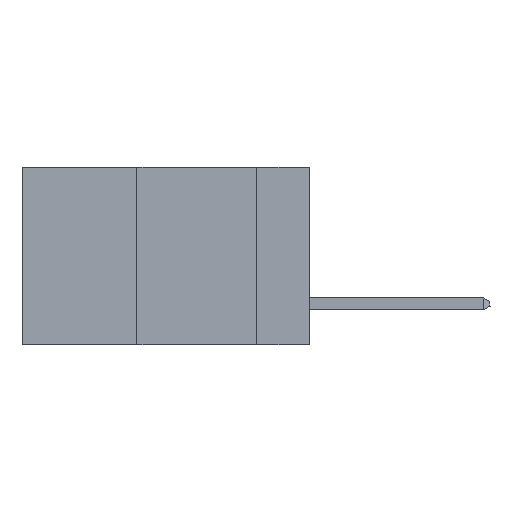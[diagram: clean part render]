
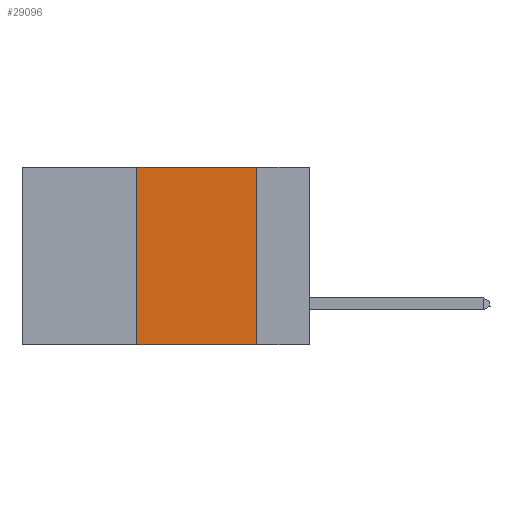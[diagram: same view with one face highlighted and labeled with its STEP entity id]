
A CAD part, left-side view. The second image highlights one B-rep face of the part: STEP entity #29096.
In plain terms, the highlighted planar face has unit normal (-1, 0, 0).
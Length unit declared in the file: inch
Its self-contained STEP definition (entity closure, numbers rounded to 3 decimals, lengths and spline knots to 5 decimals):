
#1402 = EDGE_CURVE ( 'NONE', #20306, #33130, #24977, .T. ) ;
#2687 = DIRECTION ( 'NONE',  ( 0., -1., 0. ) ) ;
#3261 = DIRECTION ( 'NONE',  ( 0., 0., -1. ) ) ;
#4467 = CARTESIAN_POINT ( 'NONE',  ( 0., 0.6, -0.37 ) ) ;
#5915 = LINE ( 'NONE', #4467, #28246 ) ;
#6120 = DIRECTION ( 'NONE',  ( 0., 0., -1. ) ) ;
#7145 = LINE ( 'NONE', #32091, #14701 ) ;
#8075 = CARTESIAN_POINT ( 'NONE',  ( 0., 0.11, 0. ) ) ;
#10261 = EDGE_CURVE ( 'NONE', #24344, #13045, #31900, .T. ) ;
#11046 = PLANE ( 'NONE',  #16051 ) ;
#11651 = EDGE_LOOP ( 'NONE', ( #13839, #12086, #23158, #34180 ) ) ;
#12086 = ORIENTED_EDGE ( 'NONE', *, *, #29518, .F. ) ;
#13045 = VERTEX_POINT ( 'NONE', #20430 ) ;
#13839 = ORIENTED_EDGE ( 'NONE', *, *, #1402, .F. ) ;
#14701 = VECTOR ( 'NONE', #31863, 39.37008 ) ;
#16051 = AXIS2_PLACEMENT_3D ( 'NONE', #24460, #32811, #6120 ) ;
#19271 = CARTESIAN_POINT ( 'NONE',  ( 0., 0.11, -0.37 ) ) ;
#20306 = VERTEX_POINT ( 'NONE', #8075 ) ;
#20430 = CARTESIAN_POINT ( 'NONE',  ( 0., 0.36, 0. ) ) ;
#20859 = DIRECTION ( 'NONE',  ( 0., 0., 1. ) ) ;
#22953 = CARTESIAN_POINT ( 'NONE',  ( 0., 0.36, -0.37 ) ) ;
#23158 = ORIENTED_EDGE ( 'NONE', *, *, #10261, .F. ) ;
#23418 = FACE_OUTER_BOUND ( 'NONE', #11651, .T. ) ;
#23602 = CARTESIAN_POINT ( 'NONE',  ( 0., 0.36, 0. ) ) ;
#24344 = VERTEX_POINT ( 'NONE', #22953 ) ;
#24460 = CARTESIAN_POINT ( 'NONE',  ( 0., 0.6, 0. ) ) ;
#24977 = LINE ( 'NONE', #30312, #30452 ) ;
#25382 = EDGE_CURVE ( 'NONE', #24344, #33130, #5915, .T. ) ;
#28246 = VECTOR ( 'NONE', #2687, 39.37008 ) ;
#29096 = ADVANCED_FACE ( 'NONE', ( #23418 ), #11046, .F. ) ;
#29518 = EDGE_CURVE ( 'NONE', #13045, #20306, #7145, .T. ) ;
#30312 = CARTESIAN_POINT ( 'NONE',  ( 0., 0.11, 0. ) ) ;
#30452 = VECTOR ( 'NONE', #3261, 39.37008 ) ;
#31863 = DIRECTION ( 'NONE',  ( 0., -1., 0. ) ) ;
#31900 = LINE ( 'NONE', #23602, #34868 ) ;
#32091 = CARTESIAN_POINT ( 'NONE',  ( 0., 0.6, 0. ) ) ;
#32811 = DIRECTION ( 'NONE',  ( 1., 0., 0. ) ) ;
#33130 = VERTEX_POINT ( 'NONE', #19271 ) ;
#34180 = ORIENTED_EDGE ( 'NONE', *, *, #25382, .T. ) ;
#34868 = VECTOR ( 'NONE', #20859, 39.37008 ) ;
